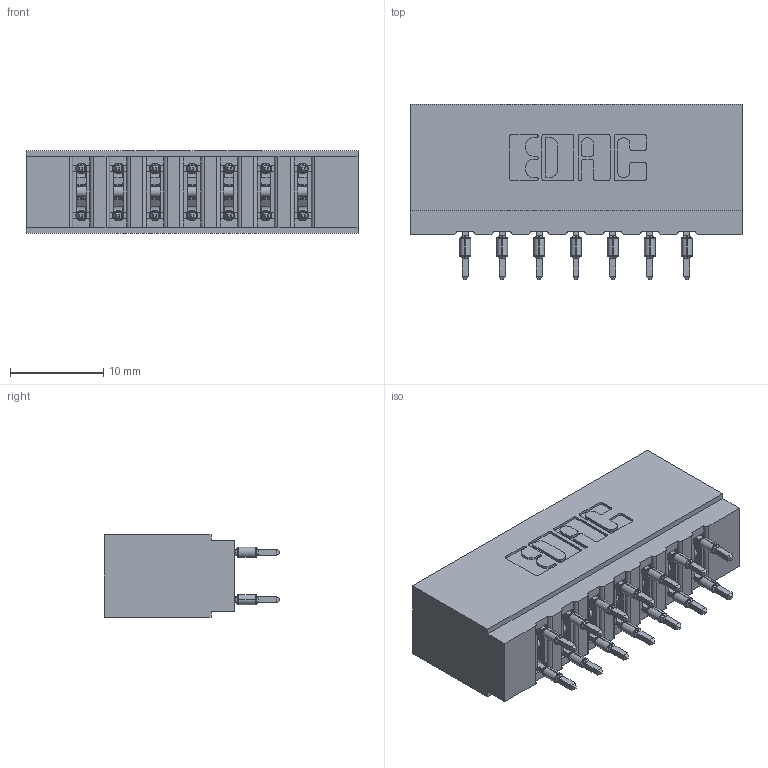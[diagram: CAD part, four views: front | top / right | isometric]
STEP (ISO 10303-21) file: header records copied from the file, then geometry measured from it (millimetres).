
FILE_DESCRIPTION (( 'STEP AP203' ), '1' );
FILE_NAME ('717-014-560-201.STEP', '2026-02-20T17:04:21', ( '' ), ( '' ), 'SwSTEP 2.0', 'SolidWorks 2023', '' );
FILE_SCHEMA (( 'CONFIG_CONTROL_DESIGN' ));
Length unit declared in the file: millimetre
Products named in the file (3): 717 Part_Insulator Option - 06; 745-292-001_560; 717-014-560-201
Assembly tree (15 placements, depth 2):
  717-014-560-201
    717 Part_Insulator Option - 06
    745-292-001_560  x14
Bounding box: 35.61 x 18.78 x 8.89 mm (x, y, z)
Volume: 3282.2 mm3; surface area: 4797.1 mm2
Topology: 15 solids, 15 shells, 1480 faces, 4045 edges, 2574 vertices
Faces by surface type: plane 775, cylinder 341, bspline 280, torus 84
Entity records: 17048 total; most frequent: CARTESIAN_POINT 3473, ORIENTED_EDGE 2838, DIRECTION 2515, EDGE_CURVE 1419, LINE 1187, VECTOR 1187, VERTEX_POINT 910, AXIS2_PLACEMENT_3D 664
